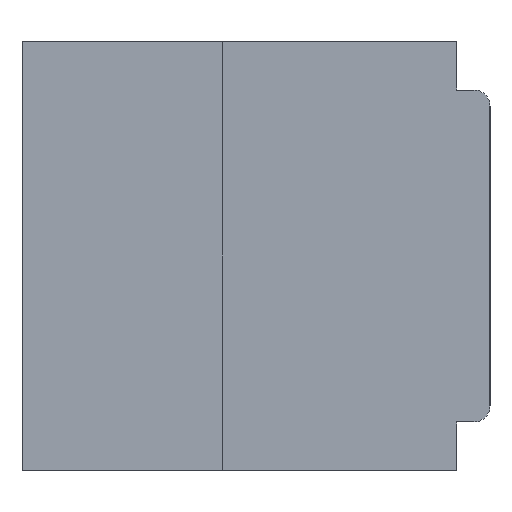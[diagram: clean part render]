
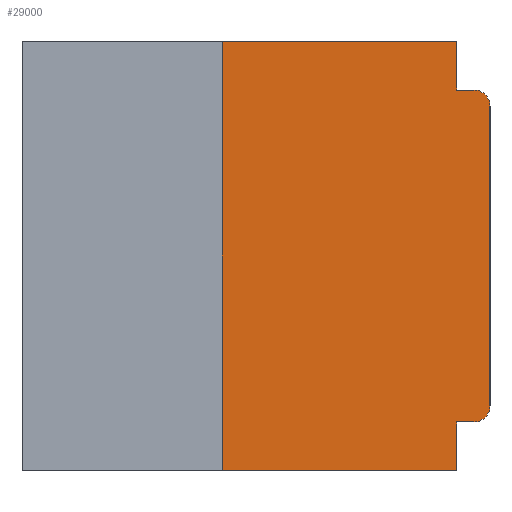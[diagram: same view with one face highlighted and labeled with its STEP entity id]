
A CAD part, left-side view. The second image highlights one B-rep face of the part: STEP entity #29000.
In plain terms, the highlighted planar face has unit normal (-1, 0, 0).
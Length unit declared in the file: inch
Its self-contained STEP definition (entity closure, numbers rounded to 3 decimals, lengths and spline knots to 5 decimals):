
#223 = CARTESIAN_POINT ( 'NONE',  ( 0., 0.031, -0.4 ) ) ;
#2003 = CIRCLE ( 'NONE', #22503, 0.015 ) ;
#3768 = ORIENTED_EDGE ( 'NONE', *, *, #4636, .T. ) ;
#3856 = DIRECTION ( 'NONE',  ( 0., 0., 1. ) ) ;
#3899 = VERTEX_POINT ( 'NONE', #42533 ) ;
#3937 = EDGE_CURVE ( 'NONE', #40474, #3899, #33232, .T. ) ;
#4609 = VERTEX_POINT ( 'NONE', #35079 ) ;
#4636 = EDGE_CURVE ( 'NONE', #48050, #20489, #42948, .T. ) ;
#4953 = VERTEX_POINT ( 'NONE', #12098 ) ;
#5146 = CARTESIAN_POINT ( 'NONE',  ( 0., 0.031, 0. ) ) ;
#6214 = PLANE ( 'NONE',  #50784 ) ;
#6465 = CARTESIAN_POINT ( 'NONE',  ( 0., 0.015, -0.355 ) ) ;
#6586 = CARTESIAN_POINT ( 'NONE',  ( 0., 0., -0.045 ) ) ;
#6981 = CARTESIAN_POINT ( 'NONE',  ( 0., 0.015, -0.34 ) ) ;
#7775 = DIRECTION ( 'NONE',  ( 0., 1., 0. ) ) ;
#9388 = ORIENTED_EDGE ( 'NONE', *, *, #23457, .T. ) ;
#10373 = ORIENTED_EDGE ( 'NONE', *, *, #15573, .T. ) ;
#10935 = EDGE_CURVE ( 'NONE', #17923, #42721, #21639, .T. ) ;
#10950 = DIRECTION ( 'NONE',  ( 0., 0., -1. ) ) ;
#11345 = LINE ( 'NONE', #17960, #32187 ) ;
#12098 = CARTESIAN_POINT ( 'NONE',  ( 0., 0.25, 0. ) ) ;
#12460 = ORIENTED_EDGE ( 'NONE', *, *, #19978, .F. ) ;
#14152 = LINE ( 'NONE', #223, #24646 ) ;
#14180 = DIRECTION ( 'NONE',  ( 1., 0., 0. ) ) ;
#14619 = DIRECTION ( 'NONE',  ( -1., 0., 0. ) ) ;
#15060 = AXIS2_PLACEMENT_3D ( 'NONE', #38000, #14619, #41950 ) ;
#15209 = CARTESIAN_POINT ( 'NONE',  ( 0., 0.25, -0.4 ) ) ;
#15304 = EDGE_CURVE ( 'NONE', #3899, #4609, #14152, .T. ) ;
#15573 = EDGE_CURVE ( 'NONE', #20489, #42721, #31865, .T. ) ;
#15893 = CARTESIAN_POINT ( 'NONE',  ( 0., 0.437, -0.4 ) ) ;
#17089 = CARTESIAN_POINT ( 'NONE',  ( 0., 0.015, -0.045 ) ) ;
#17923 = VERTEX_POINT ( 'NONE', #38097 ) ;
#17960 = CARTESIAN_POINT ( 'NONE',  ( 0., 0.031, 0. ) ) ;
#18007 = ORIENTED_EDGE ( 'NONE', *, *, #3937, .F. ) ;
#18036 = CARTESIAN_POINT ( 'NONE',  ( 0., 0.437, 0. ) ) ;
#18185 = EDGE_LOOP ( 'NONE', ( #3768, #10373, #28790, #12460, #41771, #29640, #9388, #29469, #18007, #36240 ) ) ;
#19258 = EDGE_CURVE ( 'NONE', #40474, #48050, #2003, .T. ) ;
#19978 = EDGE_CURVE ( 'NONE', #39566, #17923, #11345, .T. ) ;
#20145 = EDGE_CURVE ( 'NONE', #22833, #4953, #44414, .T. ) ;
#20489 = VERTEX_POINT ( 'NONE', #24766 ) ;
#21511 = LINE ( 'NONE', #15893, #30582 ) ;
#21639 = LINE ( 'NONE', #6586, #39835 ) ;
#22503 = AXIS2_PLACEMENT_3D ( 'NONE', #6981, #34372, #10950 ) ;
#22833 = VERTEX_POINT ( 'NONE', #15209 ) ;
#23457 = EDGE_CURVE ( 'NONE', #22833, #4609, #21511, .T. ) ;
#23672 = VECTOR ( 'NONE', #30687, 39.37008 ) ;
#24646 = VECTOR ( 'NONE', #31726, 39.37008 ) ;
#24766 = CARTESIAN_POINT ( 'NONE',  ( 0., 0., -0.06 ) ) ;
#26257 = DIRECTION ( 'NONE',  ( 0., -1., 0. ) ) ;
#26829 = CARTESIAN_POINT ( 'NONE',  ( 0., 0.25, -0.4 ) ) ;
#27997 = FACE_OUTER_BOUND ( 'NONE', #18185, .T. ) ;
#28790 = ORIENTED_EDGE ( 'NONE', *, *, #10935, .F. ) ;
#29000 = ADVANCED_FACE ( 'NONE', ( #27997 ), #6214, .F. ) ;
#29469 = ORIENTED_EDGE ( 'NONE', *, *, #15304, .F. ) ;
#29640 = ORIENTED_EDGE ( 'NONE', *, *, #20145, .F. ) ;
#30574 = EDGE_CURVE ( 'NONE', #4953, #39566, #47426, .T. ) ;
#30582 = VECTOR ( 'NONE', #47186, 39.37008 ) ;
#30687 = DIRECTION ( 'NONE',  ( 0., 0., 1. ) ) ;
#31260 = CARTESIAN_POINT ( 'NONE',  ( 0., 0., -0.355 ) ) ;
#31726 = DIRECTION ( 'NONE',  ( 0., 0., -1. ) ) ;
#31865 = CIRCLE ( 'NONE', #15060, 0.015 ) ;
#32172 = DIRECTION ( 'NONE',  ( 0., -1., 0. ) ) ;
#32187 = VECTOR ( 'NONE', #45247, 39.37008 ) ;
#32559 = VECTOR ( 'NONE', #3856, 39.37008 ) ;
#33232 = LINE ( 'NONE', #31260, #44893 ) ;
#34372 = DIRECTION ( 'NONE',  ( -1., 0., 0. ) ) ;
#35079 = CARTESIAN_POINT ( 'NONE',  ( 0., 0.031, -0.4 ) ) ;
#36240 = ORIENTED_EDGE ( 'NONE', *, *, #19258, .T. ) ;
#38000 = CARTESIAN_POINT ( 'NONE',  ( 0., 0.015, -0.06 ) ) ;
#38097 = CARTESIAN_POINT ( 'NONE',  ( 0., 0.031, -0.045 ) ) ;
#39566 = VERTEX_POINT ( 'NONE', #5146 ) ;
#39835 = VECTOR ( 'NONE', #26257, 39.37008 ) ;
#40474 = VERTEX_POINT ( 'NONE', #6465 ) ;
#41517 = DIRECTION ( 'NONE',  ( 0., 0., -1. ) ) ;
#41771 = ORIENTED_EDGE ( 'NONE', *, *, #30574, .F. ) ;
#41950 = DIRECTION ( 'NONE',  ( 0., 0., -1. ) ) ;
#42533 = CARTESIAN_POINT ( 'NONE',  ( 0., 0.031, -0.355 ) ) ;
#42721 = VERTEX_POINT ( 'NONE', #17089 ) ;
#42948 = LINE ( 'NONE', #46943, #32559 ) ;
#44414 = LINE ( 'NONE', #26829, #23672 ) ;
#44893 = VECTOR ( 'NONE', #7775, 39.37008 ) ;
#45247 = DIRECTION ( 'NONE',  ( 0., 0., -1. ) ) ;
#46188 = VECTOR ( 'NONE', #32172, 39.37008 ) ;
#46943 = CARTESIAN_POINT ( 'NONE',  ( 0., 0., 0. ) ) ;
#47186 = DIRECTION ( 'NONE',  ( 0., -1., 0. ) ) ;
#47426 = LINE ( 'NONE', #47769, #46188 ) ;
#47721 = CARTESIAN_POINT ( 'NONE',  ( 0., 0., -0.34 ) ) ;
#47769 = CARTESIAN_POINT ( 'NONE',  ( 0., 0.437, 0. ) ) ;
#48050 = VERTEX_POINT ( 'NONE', #47721 ) ;
#50784 = AXIS2_PLACEMENT_3D ( 'NONE', #18036, #14180, #41517 ) ;
